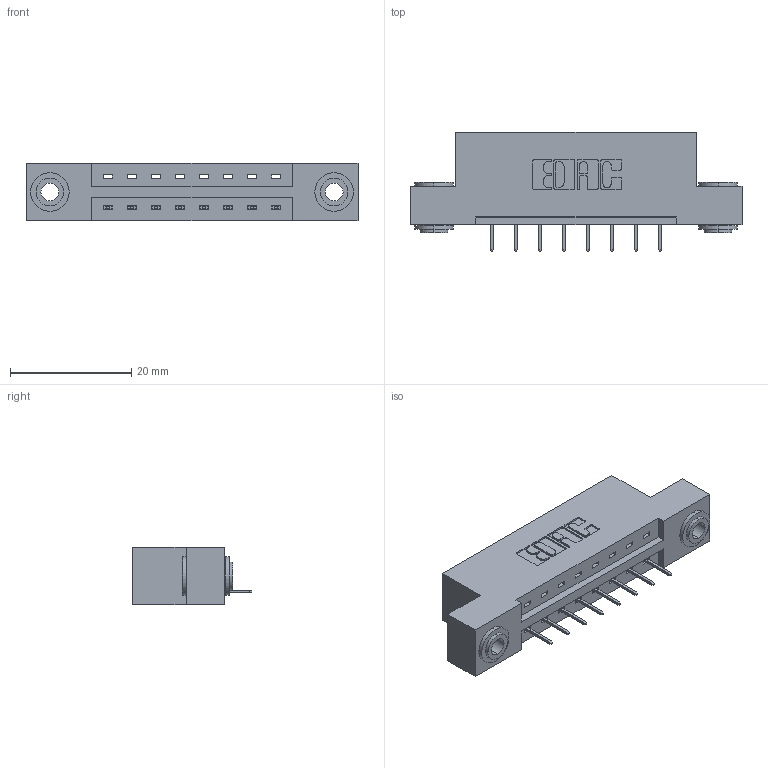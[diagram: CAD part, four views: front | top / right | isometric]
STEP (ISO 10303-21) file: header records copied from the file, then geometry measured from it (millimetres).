
FILE_DESCRIPTION (( 'STEP AP203' ), '1' );
FILE_NAME ('387-008-524-103.STEP', '2018-09-10T04:10:52', ( '' ), ( '' ), 'SwSTEP 2.0', 'SolidWorks 2016', '' );
FILE_SCHEMA (( 'CONFIG_CONTROL_DESIGN' ));
Length unit declared in the file: inch
Products named in the file (4): 337 Part_Flush Mounting Lugs - 0.156 Dia-TH; 345-292-001_345-293-124; 345-250-002_345-250-002-102; 387-008-524-103
Assembly tree (11 placements, depth 2):
  387-008-524-103
    337 Part_Flush Mounting Lugs - 0.156 Dia-TH
    345-292-001_345-293-124  x8
    345-250-002_345-250-002-102  x2
Bounding box: 54.71 x 19.69 x 9.4 mm (x, y, z)
Volume: 5248.7 mm3; surface area: 5356.6 mm2
Topology: 11 solids, 11 shells, 680 faces, 1923 edges, 1246 vertices
Faces by surface type: plane 496, cylinder 176, cone 8
Entity records: 11068 total; most frequent: CARTESIAN_POINT 1901, ORIENTED_EDGE 1838, DIRECTION 1705, EDGE_CURVE 919, LINE 771, VECTOR 771, VERTEX_POINT 606, AXIS2_PLACEMENT_3D 467
